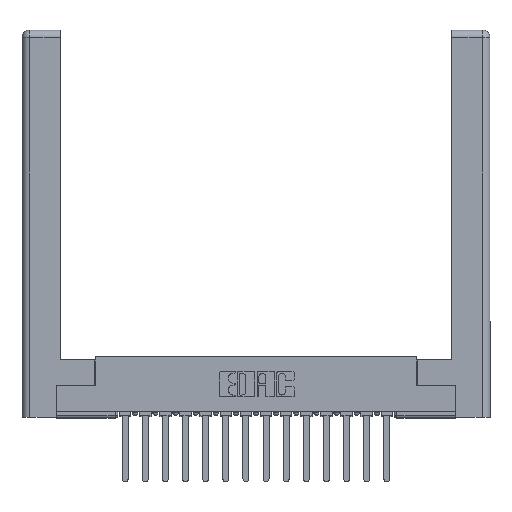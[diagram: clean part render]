
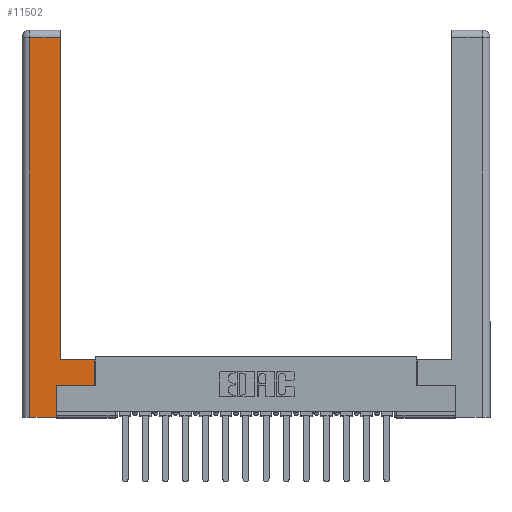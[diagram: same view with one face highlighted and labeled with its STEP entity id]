
A CAD part, top view. The second image highlights one B-rep face of the part: STEP entity #11502.
In plain terms, the highlighted planar face has unit normal (0, 0, 1).
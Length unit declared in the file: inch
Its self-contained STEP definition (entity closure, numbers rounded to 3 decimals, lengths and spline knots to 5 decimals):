
#225 = ORIENTED_EDGE ( 'NONE', *, *, #11167, .T. ) ;
#248 = DIRECTION ( 'NONE',  ( -1., 0., 0. ) ) ;
#543 = VECTOR ( 'NONE', #11113, 39.37008 ) ;
#671 = ORIENTED_EDGE ( 'NONE', *, *, #17777, .T. ) ;
#1031 = CARTESIAN_POINT ( 'NONE',  ( 0.265, 0.245, 0. ) ) ;
#1528 = VECTOR ( 'NONE', #7782, 39.37008 ) ;
#1686 = FACE_OUTER_BOUND ( 'NONE', #5034, .T. ) ;
#1794 = CARTESIAN_POINT ( 'NONE',  ( 0.265, 0.245, 0. ) ) ;
#2535 = CARTESIAN_POINT ( 'NONE',  ( 0.0615, 0., 0. ) ) ;
#2704 = DIRECTION ( 'NONE',  ( -1., 0., 0. ) ) ;
#3169 = VECTOR ( 'NONE', #13017, 39.37008 ) ;
#3563 = EDGE_CURVE ( 'NONE', #15114, #11237, #17386, .T. ) ;
#3977 = LINE ( 'NONE', #2535, #3169 ) ;
#4049 = CARTESIAN_POINT ( 'NONE',  ( 0.295, 0.45, 0. ) ) ;
#4725 = PLANE ( 'NONE',  #6496 ) ;
#4748 = LINE ( 'NONE', #1794, #7067 ) ;
#5034 = EDGE_LOOP ( 'NONE', ( #18199, #14004, #11316, #671, #225, #11992, #8797, #6273 ) ) ;
#6273 = ORIENTED_EDGE ( 'NONE', *, *, #18115, .T. ) ;
#6364 = LINE ( 'NONE', #15030, #1528 ) ;
#6369 = EDGE_CURVE ( 'NONE', #11626, #6888, #6364, .T. ) ;
#6433 = VERTEX_POINT ( 'NONE', #1031 ) ;
#6448 = CARTESIAN_POINT ( 'NONE',  ( 0.265, 0., 0. ) ) ;
#6496 = AXIS2_PLACEMENT_3D ( 'NONE', #15093, #9173, #248 ) ;
#6623 = CARTESIAN_POINT ( 'NONE',  ( 0.565, 0.245, 0. ) ) ;
#6640 = VERTEX_POINT ( 'NONE', #10043 ) ;
#6803 = DIRECTION ( 'NONE',  ( 1., 0., 0. ) ) ;
#6828 = LINE ( 'NONE', #18356, #543 ) ;
#6888 = VERTEX_POINT ( 'NONE', #9363 ) ;
#7067 = VECTOR ( 'NONE', #10440, 39.37008 ) ;
#7782 = DIRECTION ( 'NONE',  ( 0., 1., 0. ) ) ;
#7847 = CARTESIAN_POINT ( 'NONE',  ( 0.0615, 0., 0. ) ) ;
#8325 = VERTEX_POINT ( 'NONE', #6448 ) ;
#8797 = ORIENTED_EDGE ( 'NONE', *, *, #6369, .T. ) ;
#9173 = DIRECTION ( 'NONE',  ( 0., 0., -1. ) ) ;
#9285 = CARTESIAN_POINT ( 'NONE',  ( 0.0615, 2.94, 0. ) ) ;
#9363 = CARTESIAN_POINT ( 'NONE',  ( 0.565, 0.45, 0. ) ) ;
#9634 = VECTOR ( 'NONE', #10727, 39.37008 ) ;
#9833 = DIRECTION ( 'NONE',  ( 0., 1., 0. ) ) ;
#10043 = CARTESIAN_POINT ( 'NONE',  ( 0.0615, 2.94, 0. ) ) ;
#10440 = DIRECTION ( 'NONE',  ( 0., 1., 0. ) ) ;
#10727 = DIRECTION ( 'NONE',  ( -1., 0., 0. ) ) ;
#11113 = DIRECTION ( 'NONE',  ( 1., 0., 0. ) ) ;
#11167 = EDGE_CURVE ( 'NONE', #8325, #6433, #4748, .T. ) ;
#11237 = VERTEX_POINT ( 'NONE', #15489 ) ;
#11316 = ORIENTED_EDGE ( 'NONE', *, *, #14552, .T. ) ;
#11502 = ADVANCED_FACE ( 'NONE', ( #1686 ), #4725, .F. ) ;
#11626 = VERTEX_POINT ( 'NONE', #6623 ) ;
#11768 = EDGE_CURVE ( 'NONE', #6433, #11626, #18332, .T. ) ;
#11992 = ORIENTED_EDGE ( 'NONE', *, *, #11768, .T. ) ;
#12710 = LINE ( 'NONE', #4049, #15451 ) ;
#13017 = DIRECTION ( 'NONE',  ( 0., -1., 0. ) ) ;
#13603 = LINE ( 'NONE', #9285, #9634 ) ;
#14004 = ORIENTED_EDGE ( 'NONE', *, *, #17573, .T. ) ;
#14043 = CARTESIAN_POINT ( 'NONE',  ( 0.565, 0.245, 0. ) ) ;
#14552 = EDGE_CURVE ( 'NONE', #6640, #14718, #3977, .T. ) ;
#14718 = VERTEX_POINT ( 'NONE', #7847 ) ;
#15030 = CARTESIAN_POINT ( 'NONE',  ( 0.565, 0.45, 0. ) ) ;
#15093 = CARTESIAN_POINT ( 'NONE',  ( 0., 0., 0. ) ) ;
#15114 = VERTEX_POINT ( 'NONE', #15271 ) ;
#15271 = CARTESIAN_POINT ( 'NONE',  ( 0.295, 0.45, 0. ) ) ;
#15451 = VECTOR ( 'NONE', #2704, 39.37008 ) ;
#15489 = CARTESIAN_POINT ( 'NONE',  ( 0.295, 2.94, 0. ) ) ;
#15571 = CARTESIAN_POINT ( 'NONE',  ( 0.295, 3., 0. ) ) ;
#17386 = LINE ( 'NONE', #15571, #18209 ) ;
#17430 = VECTOR ( 'NONE', #6803, 39.37008 ) ;
#17573 = EDGE_CURVE ( 'NONE', #11237, #6640, #13603, .T. ) ;
#17777 = EDGE_CURVE ( 'NONE', #14718, #8325, #6828, .T. ) ;
#18115 = EDGE_CURVE ( 'NONE', #6888, #15114, #12710, .T. ) ;
#18199 = ORIENTED_EDGE ( 'NONE', *, *, #3563, .T. ) ;
#18209 = VECTOR ( 'NONE', #9833, 39.37008 ) ;
#18332 = LINE ( 'NONE', #14043, #17430 ) ;
#18356 = CARTESIAN_POINT ( 'NONE',  ( 0.265, 0., 0. ) ) ;
